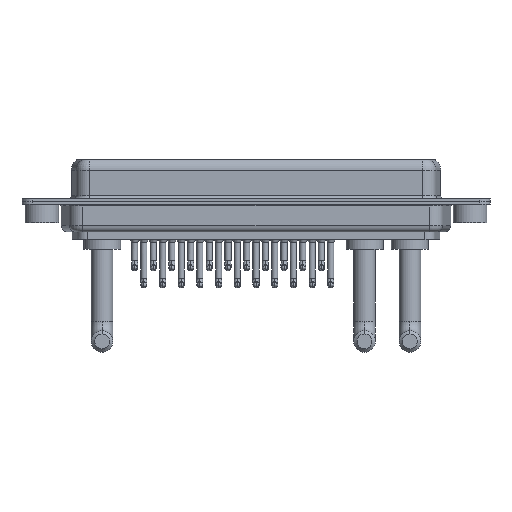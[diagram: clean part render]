
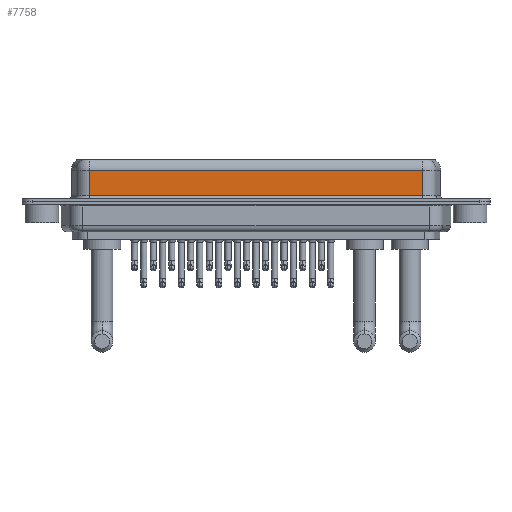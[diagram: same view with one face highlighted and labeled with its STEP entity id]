
A CAD part, front view. The second image highlights one B-rep face of the part: STEP entity #7758.
In plain terms, the highlighted planar face has unit normal (0, -1, 0).
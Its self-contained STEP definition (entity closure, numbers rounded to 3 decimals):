
#231 = CARTESIAN_POINT ( 'NONE',  ( 56.462, -3.95, 6.4 ) ) ;
#1368 = LINE ( 'NONE', #23383, #1750 ) ;
#1750 = VECTOR ( 'NONE', #6871, 1000. ) ;
#2580 = VERTEX_POINT ( 'NONE', #4440 ) ;
#2943 = VERTEX_POINT ( 'NONE', #18402 ) ;
#3104 = FACE_OUTER_BOUND ( 'NONE', #13768, .T. ) ;
#3269 = CARTESIAN_POINT ( 'NONE',  ( 7.038, -3.95, 6.4 ) ) ;
#4440 = CARTESIAN_POINT ( 'NONE',  ( 7.038, -3.95, 4.65 ) ) ;
#4895 = PLANE ( 'NONE',  #12575 ) ;
#4955 = LINE ( 'NONE', #3269, #19169 ) ;
#5617 = EDGE_CURVE ( 'NONE', #7040, #2943, #1368, .T. ) ;
#5671 = ORIENTED_EDGE ( 'NONE', *, *, #19968, .T. ) ;
#6580 = CARTESIAN_POINT ( 'NONE',  ( 56.462, -3.95, 4.65 ) ) ;
#6670 = DIRECTION ( 'NONE',  ( 0., 1., 0. ) ) ;
#6871 = DIRECTION ( 'NONE',  ( 1., 0., 0. ) ) ;
#7040 = VERTEX_POINT ( 'NONE', #10097 ) ;
#7097 = DIRECTION ( 'NONE',  ( 0., 0., -1. ) ) ;
#7758 = ADVANCED_FACE ( 'NONE', ( #3104 ), #4895, .F. ) ;
#10097 = CARTESIAN_POINT ( 'NONE',  ( 7.038, -3.95, 0.9 ) ) ;
#10232 = EDGE_CURVE ( 'NONE', #2580, #7040, #4955, .T. ) ;
#12575 = AXIS2_PLACEMENT_3D ( 'NONE', #15967, #6670, #17417 ) ;
#13768 = EDGE_LOOP ( 'NONE', ( #15175, #5671, #14695, #16589 ) ) ;
#14313 = LINE ( 'NONE', #23348, #22196 ) ;
#14537 = LINE ( 'NONE', #231, #18832 ) ;
#14695 = ORIENTED_EDGE ( 'NONE', *, *, #10232, .T. ) ;
#14903 = DIRECTION ( 'NONE',  ( 0., 0., -1. ) ) ;
#15175 = ORIENTED_EDGE ( 'NONE', *, *, #23684, .F. ) ;
#15967 = CARTESIAN_POINT ( 'NONE',  ( 56.462, -3.95, 6.4 ) ) ;
#16589 = ORIENTED_EDGE ( 'NONE', *, *, #5617, .T. ) ;
#17417 = DIRECTION ( 'NONE',  ( 0., 0., 1. ) ) ;
#17454 = DIRECTION ( 'NONE',  ( -1., 0., 0. ) ) ;
#18402 = CARTESIAN_POINT ( 'NONE',  ( 56.462, -3.95, 0.9 ) ) ;
#18832 = VECTOR ( 'NONE', #14903, 1000. ) ;
#19169 = VECTOR ( 'NONE', #7097, 1000. ) ;
#19968 = EDGE_CURVE ( 'NONE', #23536, #2580, #14313, .T. ) ;
#22196 = VECTOR ( 'NONE', #17454, 1000. ) ;
#23348 = CARTESIAN_POINT ( 'NONE',  ( 56.462, -3.95, 4.65 ) ) ;
#23383 = CARTESIAN_POINT ( 'NONE',  ( 56.462, -3.95, 0.9 ) ) ;
#23536 = VERTEX_POINT ( 'NONE', #6580 ) ;
#23684 = EDGE_CURVE ( 'NONE', #23536, #2943, #14537, .T. ) ;
